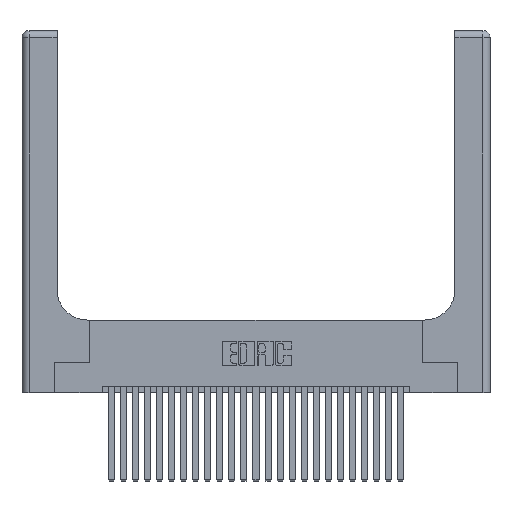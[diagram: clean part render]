
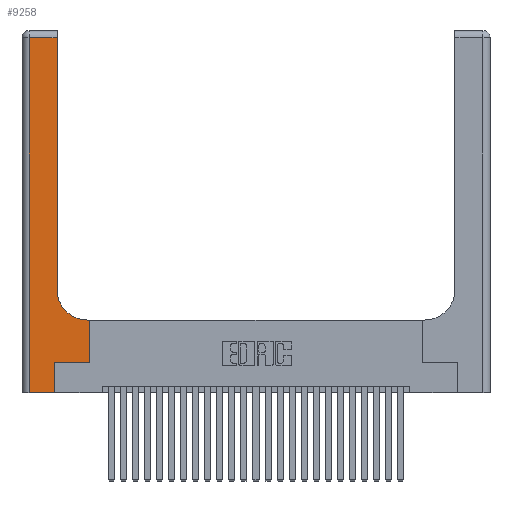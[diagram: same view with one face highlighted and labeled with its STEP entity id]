
A CAD part, top view. The second image highlights one B-rep face of the part: STEP entity #9258.
In plain terms, the highlighted planar face has unit normal (0, 0, 1).
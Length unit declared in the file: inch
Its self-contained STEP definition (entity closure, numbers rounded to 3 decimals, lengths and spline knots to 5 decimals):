
#450 = DIRECTION ( 'NONE',  ( 0., 1., 0. ) ) ;
#1403 = CARTESIAN_POINT ( 'NONE',  ( 0.5585, 0.6, 0.37 ) ) ;
#1967 = DIRECTION ( 'NONE',  ( 1., 0., 0. ) ) ;
#2059 = CARTESIAN_POINT ( 'NONE',  ( 0.269, 0.25, 0.37 ) ) ;
#2106 = VERTEX_POINT ( 'NONE', #2357 ) ;
#2115 = EDGE_CURVE ( 'NONE', #22606, #21310, #22078, .T. ) ;
#2357 = CARTESIAN_POINT ( 'NONE',  ( 0.06, 2.94, 0.37 ) ) ;
#2946 = CARTESIAN_POINT ( 'NONE',  ( 0.2915, 0.6, 0.37 ) ) ;
#3211 = VERTEX_POINT ( 'NONE', #5345 ) ;
#4297 = CARTESIAN_POINT ( 'NONE',  ( 0.269, 0., 0.37 ) ) ;
#4461 = EDGE_LOOP ( 'NONE', ( #9189, #22082, #22611, #12549, #16441, #15676, #15622, #8199, #11503 ) ) ;
#4659 = CARTESIAN_POINT ( 'NONE',  ( 0.2915, 3., 0.37 ) ) ;
#4943 = DIRECTION ( 'NONE',  ( 1., 0., 0. ) ) ;
#5345 = CARTESIAN_POINT ( 'NONE',  ( 0.2915, 2.94, 0.37 ) ) ;
#5530 = LINE ( 'NONE', #11041, #21337 ) ;
#6558 = DIRECTION ( 'NONE',  ( 0., 0., -1. ) ) ;
#6660 = VECTOR ( 'NONE', #18240, 39.37008 ) ;
#6751 = EDGE_CURVE ( 'NONE', #2106, #20321, #11531, .T. ) ;
#7176 = AXIS2_PLACEMENT_3D ( 'NONE', #8070, #22547, #10163 ) ;
#8070 = CARTESIAN_POINT ( 'NONE',  ( 0., 3., 0.37 ) ) ;
#8199 = ORIENTED_EDGE ( 'NONE', *, *, #19563, .T. ) ;
#9189 = ORIENTED_EDGE ( 'NONE', *, *, #10576, .T. ) ;
#9248 = CARTESIAN_POINT ( 'NONE',  ( 0.06, 0., 0.37 ) ) ;
#9253 = CARTESIAN_POINT ( 'NONE',  ( 0.5415, 0.6, 0.37 ) ) ;
#9258 = ADVANCED_FACE ( 'NONE', ( #14046 ), #18286, .F. ) ;
#10163 = DIRECTION ( 'NONE',  ( -1., 0., 0. ) ) ;
#10377 = LINE ( 'NONE', #2946, #15273 ) ;
#10576 = EDGE_CURVE ( 'NONE', #15833, #3211, #12994, .T. ) ;
#11041 = CARTESIAN_POINT ( 'NONE',  ( 0., 0., 0.37 ) ) ;
#11044 = EDGE_CURVE ( 'NONE', #16416, #22606, #23986, .T. ) ;
#11114 = VECTOR ( 'NONE', #1967, 39.37008 ) ;
#11503 = ORIENTED_EDGE ( 'NONE', *, *, #25020, .T. ) ;
#11531 = LINE ( 'NONE', #24518, #6660 ) ;
#12549 = ORIENTED_EDGE ( 'NONE', *, *, #19527, .T. ) ;
#12847 = CARTESIAN_POINT ( 'NONE',  ( 0.269, 0.25, 0.37 ) ) ;
#12994 = LINE ( 'NONE', #4659, #13646 ) ;
#13029 = CARTESIAN_POINT ( 'NONE',  ( 0.5585, 0.25, 0.37 ) ) ;
#13342 = VECTOR ( 'NONE', #14551, 39.37008 ) ;
#13646 = VECTOR ( 'NONE', #450, 39.37008 ) ;
#14046 = FACE_OUTER_BOUND ( 'NONE', #4461, .T. ) ;
#14551 = DIRECTION ( 'NONE',  ( -1., 0., 0. ) ) ;
#15273 = VECTOR ( 'NONE', #15386, 39.37008 ) ;
#15356 = AXIS2_PLACEMENT_3D ( 'NONE', #18923, #6558, #21000 ) ;
#15386 = DIRECTION ( 'NONE',  ( -1., 0., 0. ) ) ;
#15622 = ORIENTED_EDGE ( 'NONE', *, *, #22683, .T. ) ;
#15676 = ORIENTED_EDGE ( 'NONE', *, *, #2115, .T. ) ;
#15833 = VERTEX_POINT ( 'NONE', #25353 ) ;
#15871 = CIRCLE ( 'NONE', #15356, 0.25 ) ;
#16113 = CARTESIAN_POINT ( 'NONE',  ( 0., 2.94, 0.37 ) ) ;
#16191 = DIRECTION ( 'NONE',  ( 0., 1., 0. ) ) ;
#16416 = VERTEX_POINT ( 'NONE', #4297 ) ;
#16441 = ORIENTED_EDGE ( 'NONE', *, *, #11044, .T. ) ;
#16628 = CARTESIAN_POINT ( 'NONE',  ( 0.5585, 0.25, 0.37 ) ) ;
#18240 = DIRECTION ( 'NONE',  ( 0., -1., 0. ) ) ;
#18286 = PLANE ( 'NONE',  #7176 ) ;
#18760 = EDGE_CURVE ( 'NONE', #3211, #2106, #23707, .T. ) ;
#18905 = VECTOR ( 'NONE', #25451, 39.37008 ) ;
#18923 = CARTESIAN_POINT ( 'NONE',  ( 0.5415, 0.85, 0.37 ) ) ;
#19527 = EDGE_CURVE ( 'NONE', #20321, #16416, #5530, .T. ) ;
#19548 = LINE ( 'NONE', #13029, #18905 ) ;
#19563 = EDGE_CURVE ( 'NONE', #26474, #25207, #10377, .T. ) ;
#20197 = CARTESIAN_POINT ( 'NONE',  ( 0.269, 0., 0.37 ) ) ;
#20321 = VERTEX_POINT ( 'NONE', #9248 ) ;
#21000 = DIRECTION ( 'NONE',  ( 1., 0., 0. ) ) ;
#21310 = VERTEX_POINT ( 'NONE', #16628 ) ;
#21337 = VECTOR ( 'NONE', #4943, 39.37008 ) ;
#22078 = LINE ( 'NONE', #2059, #11114 ) ;
#22082 = ORIENTED_EDGE ( 'NONE', *, *, #18760, .T. ) ;
#22547 = DIRECTION ( 'NONE',  ( 0., 0., -1. ) ) ;
#22606 = VERTEX_POINT ( 'NONE', #12847 ) ;
#22611 = ORIENTED_EDGE ( 'NONE', *, *, #6751, .T. ) ;
#22683 = EDGE_CURVE ( 'NONE', #21310, #26474, #19548, .T. ) ;
#23707 = LINE ( 'NONE', #16113, #13342 ) ;
#23986 = LINE ( 'NONE', #20197, #24647 ) ;
#24518 = CARTESIAN_POINT ( 'NONE',  ( 0.06, 3., 0.37 ) ) ;
#24647 = VECTOR ( 'NONE', #16191, 39.37008 ) ;
#25020 = EDGE_CURVE ( 'NONE', #25207, #15833, #15871, .T. ) ;
#25207 = VERTEX_POINT ( 'NONE', #9253 ) ;
#25353 = CARTESIAN_POINT ( 'NONE',  ( 0.2915, 0.85, 0.37 ) ) ;
#25451 = DIRECTION ( 'NONE',  ( 0., 1., 0. ) ) ;
#26474 = VERTEX_POINT ( 'NONE', #1403 ) ;
